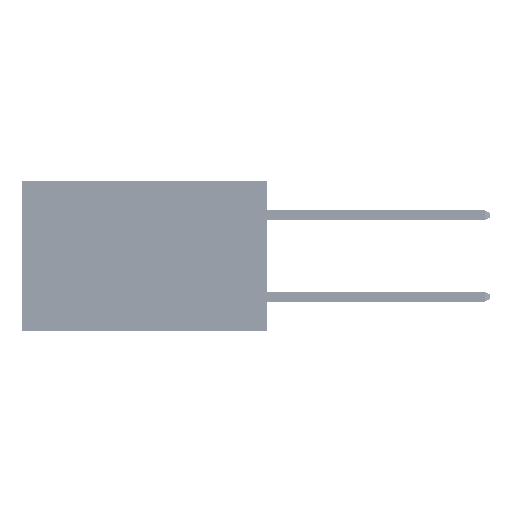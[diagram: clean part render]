
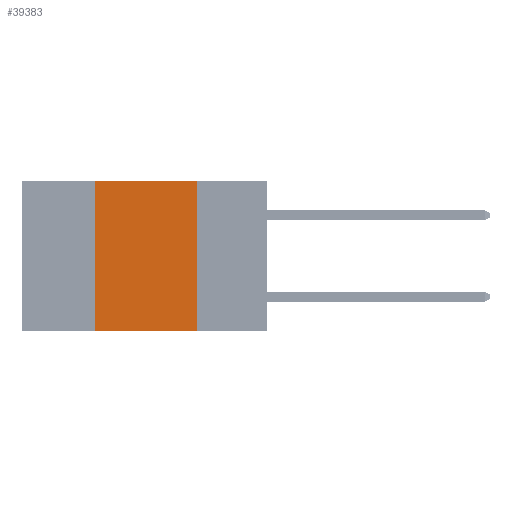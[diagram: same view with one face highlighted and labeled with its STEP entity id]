
A CAD part, left-side view. The second image highlights one B-rep face of the part: STEP entity #39383.
In plain terms, the highlighted planar face has unit normal (-1, 0, 0).
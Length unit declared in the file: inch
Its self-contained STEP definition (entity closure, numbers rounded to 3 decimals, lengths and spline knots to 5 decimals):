
#33 = VECTOR ( 'NONE', #43942, 39.37008 ) ;
#1278 = LINE ( 'NONE', #48629, #49874 ) ;
#2534 = AXIS2_PLACEMENT_3D ( 'NONE', #22704, #2981, #34560 ) ;
#2981 = DIRECTION ( 'NONE',  ( 1., 0., 0. ) ) ;
#4407 = LINE ( 'NONE', #44003, #22373 ) ;
#7930 = VERTEX_POINT ( 'NONE', #20401 ) ;
#8391 = DIRECTION ( 'NONE',  ( 0., 0., 1. ) ) ;
#8482 = ORIENTED_EDGE ( 'NONE', *, *, #11566, .F. ) ;
#10931 = VECTOR ( 'NONE', #8391, 39.37008 ) ;
#11566 = EDGE_CURVE ( 'NONE', #7930, #49747, #1278, .T. ) ;
#11946 = CARTESIAN_POINT ( 'NONE',  ( 0., 0.17, 0. ) ) ;
#12379 = CARTESIAN_POINT ( 'NONE',  ( 0., 0.6, -0.37 ) ) ;
#12986 = ORIENTED_EDGE ( 'NONE', *, *, #43473, .F. ) ;
#13026 = LINE ( 'NONE', #16399, #10931 ) ;
#13207 = DIRECTION ( 'NONE',  ( 0., -1., 0. ) ) ;
#16399 = CARTESIAN_POINT ( 'NONE',  ( 0., 0.42, 0. ) ) ;
#17807 = ORIENTED_EDGE ( 'NONE', *, *, #41144, .T. ) ;
#18805 = FACE_OUTER_BOUND ( 'NONE', #31101, .T. ) ;
#20401 = CARTESIAN_POINT ( 'NONE',  ( 0., 0.42, 0. ) ) ;
#20685 = LINE ( 'NONE', #12379, #33 ) ;
#22373 = VECTOR ( 'NONE', #31619, 39.37008 ) ;
#22704 = CARTESIAN_POINT ( 'NONE',  ( 0., 0.6, 0. ) ) ;
#29305 = CARTESIAN_POINT ( 'NONE',  ( 0., 0.17, -0.37 ) ) ;
#29916 = ORIENTED_EDGE ( 'NONE', *, *, #40552, .F. ) ;
#31101 = EDGE_LOOP ( 'NONE', ( #29916, #8482, #12986, #17807 ) ) ;
#31619 = DIRECTION ( 'NONE',  ( 0., 0., -1. ) ) ;
#34316 = VERTEX_POINT ( 'NONE', #42897 ) ;
#34560 = DIRECTION ( 'NONE',  ( 0., 0., -1. ) ) ;
#37700 = PLANE ( 'NONE',  #2534 ) ;
#39383 = ADVANCED_FACE ( 'NONE', ( #18805 ), #37700, .F. ) ;
#39616 = VERTEX_POINT ( 'NONE', #29305 ) ;
#40552 = EDGE_CURVE ( 'NONE', #49747, #39616, #4407, .T. ) ;
#41144 = EDGE_CURVE ( 'NONE', #34316, #39616, #20685, .T. ) ;
#42897 = CARTESIAN_POINT ( 'NONE',  ( 0., 0.42, -0.37 ) ) ;
#43473 = EDGE_CURVE ( 'NONE', #34316, #7930, #13026, .T. ) ;
#43942 = DIRECTION ( 'NONE',  ( 0., -1., 0. ) ) ;
#44003 = CARTESIAN_POINT ( 'NONE',  ( 0., 0.17, 0. ) ) ;
#48629 = CARTESIAN_POINT ( 'NONE',  ( 0., 0.6, 0. ) ) ;
#49747 = VERTEX_POINT ( 'NONE', #11946 ) ;
#49874 = VECTOR ( 'NONE', #13207, 39.37008 ) ;
